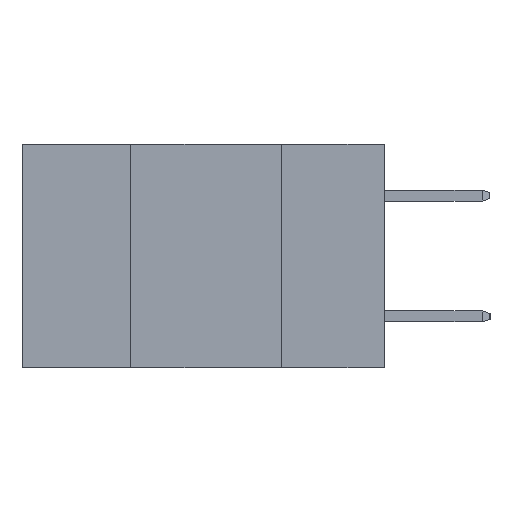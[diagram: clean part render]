
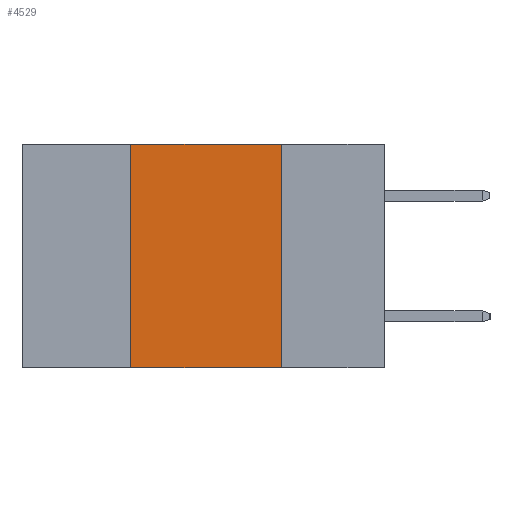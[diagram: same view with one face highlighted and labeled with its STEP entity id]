
A CAD part, left-side view. The second image highlights one B-rep face of the part: STEP entity #4529.
In plain terms, the highlighted planar face has unit normal (-1, 0, 0).
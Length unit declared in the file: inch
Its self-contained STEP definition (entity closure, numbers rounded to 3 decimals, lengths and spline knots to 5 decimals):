
#105 = VECTOR ( 'NONE', #9892, 39.37008 ) ;
#151 = VERTEX_POINT ( 'NONE', #12246 ) ;
#222 = CARTESIAN_POINT ( 'NONE',  ( 0., 0.42, 0. ) ) ;
#694 = CARTESIAN_POINT ( 'NONE',  ( 0., 0.17, 0. ) ) ;
#1284 = ORIENTED_EDGE ( 'NONE', *, *, #10065, .F. ) ;
#1430 = ORIENTED_EDGE ( 'NONE', *, *, #7301, .F. ) ;
#1558 = LINE ( 'NONE', #10459, #6634 ) ;
#2663 = LINE ( 'NONE', #9861, #105 ) ;
#3015 = ORIENTED_EDGE ( 'NONE', *, *, #11902, .F. ) ;
#4151 = DIRECTION ( 'NONE',  ( 0., 0., -1. ) ) ;
#4494 = DIRECTION ( 'NONE',  ( 0., 0., -1. ) ) ;
#4529 = ADVANCED_FACE ( 'NONE', ( #10108 ), #4762, .F. ) ;
#4645 = DIRECTION ( 'NONE',  ( 1., 0., 0. ) ) ;
#4762 = PLANE ( 'NONE',  #10665 ) ;
#5357 = VERTEX_POINT ( 'NONE', #222 ) ;
#5663 = CARTESIAN_POINT ( 'NONE',  ( 0., 0.6, 0. ) ) ;
#5840 = ORIENTED_EDGE ( 'NONE', *, *, #6199, .T. ) ;
#5933 = DIRECTION ( 'NONE',  ( 0., -1., 0. ) ) ;
#5944 = VECTOR ( 'NONE', #4151, 39.37008 ) ;
#6016 = CARTESIAN_POINT ( 'NONE',  ( 0., 0.6, -0.37 ) ) ;
#6199 = EDGE_CURVE ( 'NONE', #9386, #151, #12090, .T. ) ;
#6482 = CARTESIAN_POINT ( 'NONE',  ( 0., 0.42, -0.37 ) ) ;
#6634 = VECTOR ( 'NONE', #7568, 39.37008 ) ;
#7301 = EDGE_CURVE ( 'NONE', #9386, #5357, #2663, .T. ) ;
#7568 = DIRECTION ( 'NONE',  ( 0., -1., 0. ) ) ;
#8597 = LINE ( 'NONE', #11825, #5944 ) ;
#9386 = VERTEX_POINT ( 'NONE', #6482 ) ;
#9650 = VECTOR ( 'NONE', #5933, 39.37008 ) ;
#9861 = CARTESIAN_POINT ( 'NONE',  ( 0., 0.42, -0.37 ) ) ;
#9892 = DIRECTION ( 'NONE',  ( 0., 0., 1. ) ) ;
#9948 = EDGE_LOOP ( 'NONE', ( #3015, #1284, #1430, #5840 ) ) ;
#10065 = EDGE_CURVE ( 'NONE', #5357, #10678, #1558, .T. ) ;
#10108 = FACE_OUTER_BOUND ( 'NONE', #9948, .T. ) ;
#10459 = CARTESIAN_POINT ( 'NONE',  ( 0., 0.6, 0. ) ) ;
#10665 = AXIS2_PLACEMENT_3D ( 'NONE', #5663, #4645, #4494 ) ;
#10678 = VERTEX_POINT ( 'NONE', #694 ) ;
#11825 = CARTESIAN_POINT ( 'NONE',  ( 0., 0.17, -0.37 ) ) ;
#11902 = EDGE_CURVE ( 'NONE', #10678, #151, #8597, .T. ) ;
#12090 = LINE ( 'NONE', #6016, #9650 ) ;
#12246 = CARTESIAN_POINT ( 'NONE',  ( 0., 0.17, -0.37 ) ) ;
